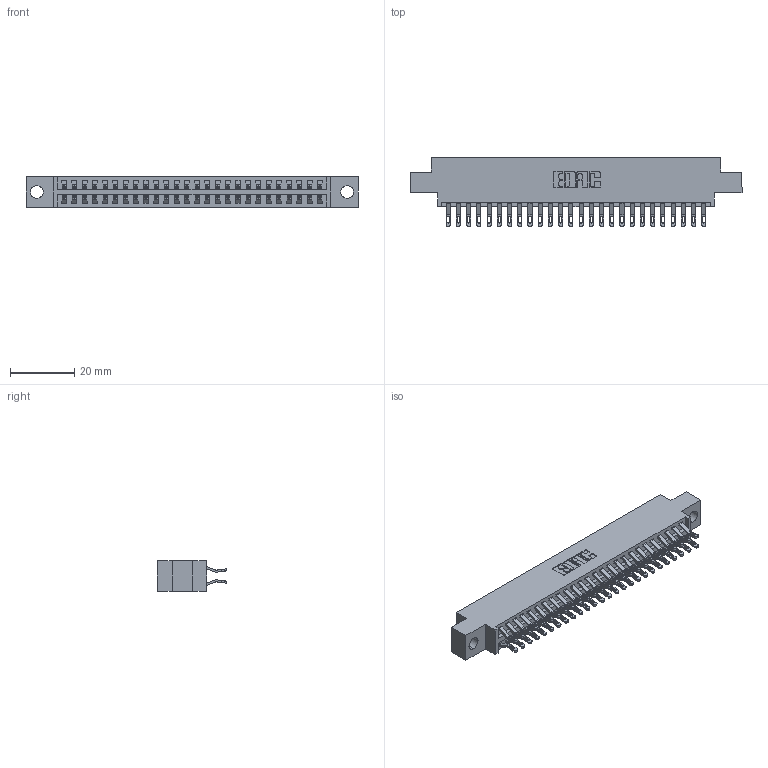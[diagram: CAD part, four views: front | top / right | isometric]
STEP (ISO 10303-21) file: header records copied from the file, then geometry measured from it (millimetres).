
FILE_DESCRIPTION (( 'STEP AP203' ), '1' );
FILE_NAME ('346-052-555-804.STEP', '2018-08-28T00:11:31', ( '' ), ( '' ), 'SwSTEP 2.0', 'SolidWorks 2016', '' );
FILE_SCHEMA (( 'CONFIG_CONTROL_DESIGN' ));
Length unit declared in the file: inch
Products named in the file (3): 345-292-001_555 Tail; 346-052-555-804; 346 Part_0.170 Offset - 0.156 Dia-TH
Assembly tree (53 placements, depth 2):
  346-052-555-804
    346 Part_0.170 Offset - 0.156 Dia-TH
    345-292-001_555 Tail  x52
Bounding box: 103.12 x 21.46 x 9.4 mm (x, y, z)
Volume: 9840 mm3; surface area: 13804.8 mm2
Topology: 53 solids, 53 shells, 3142 faces, 9857 edges, 6570 vertices
Faces by surface type: plane 1796, cylinder 1346
Entity records: 19583 total; most frequent: CARTESIAN_POINT 3286, ORIENTED_EDGE 3190, DIRECTION 2915, EDGE_CURVE 1595, LINE 1339, VECTOR 1339, VERTEX_POINT 1062, AXIS2_PLACEMENT_3D 788
